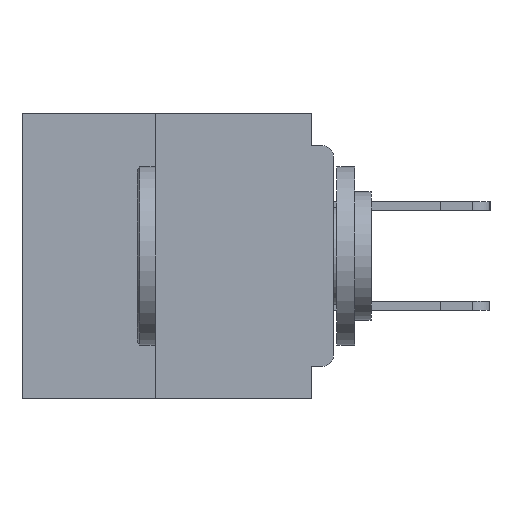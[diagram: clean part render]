
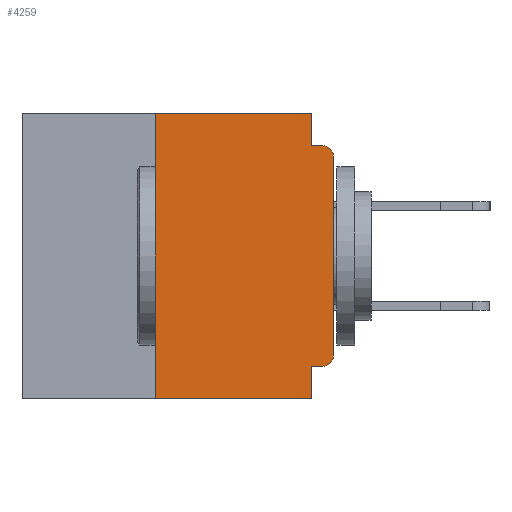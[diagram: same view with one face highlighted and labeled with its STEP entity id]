
A CAD part, left-side view. The second image highlights one B-rep face of the part: STEP entity #4259.
In plain terms, the highlighted planar face has unit normal (-1, 0, 0).
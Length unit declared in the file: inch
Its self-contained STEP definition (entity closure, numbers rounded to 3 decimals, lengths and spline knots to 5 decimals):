
#258 = AXIS2_PLACEMENT_3D ( 'NONE', #18743, #47326, #22875 ) ;
#259 = ORIENTED_EDGE ( 'NONE', *, *, #43609, .F. ) ;
#722 = DIRECTION ( 'NONE',  ( 0., 0., -1. ) ) ;
#890 = CARTESIAN_POINT ( 'NONE',  ( 0., 0.25, -0.4 ) ) ;
#1025 = LINE ( 'NONE', #19762, #39483 ) ;
#1196 = DIRECTION ( 'NONE',  ( 0., 0., -1. ) ) ;
#2159 = VERTEX_POINT ( 'NONE', #35786 ) ;
#2921 = LINE ( 'NONE', #14245, #35593 ) ;
#4256 = ORIENTED_EDGE ( 'NONE', *, *, #52456, .T. ) ;
#4259 = ADVANCED_FACE ( 'NONE', ( #37608 ), #41574, .F. ) ;
#6706 = CARTESIAN_POINT ( 'NONE',  ( 0., 0., -0.06 ) ) ;
#6852 = EDGE_CURVE ( 'NONE', #24654, #2159, #17384, .T. ) ;
#7343 = LINE ( 'NONE', #21171, #49592 ) ;
#9347 = CARTESIAN_POINT ( 'NONE',  ( 0., 0., -0.34 ) ) ;
#9559 = VERTEX_POINT ( 'NONE', #39944 ) ;
#9707 = LINE ( 'NONE', #12195, #41114 ) ;
#10303 = LINE ( 'NONE', #21649, #19936 ) ;
#10613 = EDGE_CURVE ( 'NONE', #16969, #31939, #20406, .T. ) ;
#11067 = CIRCLE ( 'NONE', #12804, 0.015 ) ;
#12195 = CARTESIAN_POINT ( 'NONE',  ( 0., 0., 0. ) ) ;
#12804 = AXIS2_PLACEMENT_3D ( 'NONE', #24137, #52662, #28261 ) ;
#14245 = CARTESIAN_POINT ( 'NONE',  ( 0., 0., -0.045 ) ) ;
#15128 = EDGE_CURVE ( 'NONE', #24654, #36146, #7343, .T. ) ;
#16969 = VERTEX_POINT ( 'NONE', #49732 ) ;
#17325 = ORIENTED_EDGE ( 'NONE', *, *, #39891, .F. ) ;
#17351 = CARTESIAN_POINT ( 'NONE',  ( 0., 0.25, -0.4 ) ) ;
#17384 = LINE ( 'NONE', #17351, #27018 ) ;
#18606 = VECTOR ( 'NONE', #28648, 39.37008 ) ;
#18615 = CARTESIAN_POINT ( 'NONE',  ( 0., 0.437, 0. ) ) ;
#18743 = CARTESIAN_POINT ( 'NONE',  ( 0., 0.015, -0.34 ) ) ;
#19762 = CARTESIAN_POINT ( 'NONE',  ( 0., 0., -0.355 ) ) ;
#19936 = VECTOR ( 'NONE', #1196, 39.37008 ) ;
#20406 = CIRCLE ( 'NONE', #258, 0.015 ) ;
#20956 = VERTEX_POINT ( 'NONE', #41401 ) ;
#21171 = CARTESIAN_POINT ( 'NONE',  ( 0., 0.437, -0.4 ) ) ;
#21241 = VERTEX_POINT ( 'NONE', #22599 ) ;
#21649 = CARTESIAN_POINT ( 'NONE',  ( 0., 0.031, 0. ) ) ;
#22599 = CARTESIAN_POINT ( 'NONE',  ( 0., 0.015, -0.045 ) ) ;
#22666 = CARTESIAN_POINT ( 'NONE',  ( 0., 0.031, -0.4 ) ) ;
#22742 = DIRECTION ( 'NONE',  ( 0., -1., 0. ) ) ;
#22875 = DIRECTION ( 'NONE',  ( 0., 0., -1. ) ) ;
#24137 = CARTESIAN_POINT ( 'NONE',  ( 0., 0.015, -0.06 ) ) ;
#24534 = CARTESIAN_POINT ( 'NONE',  ( 0., 0.031, -0.4 ) ) ;
#24654 = VERTEX_POINT ( 'NONE', #890 ) ;
#25281 = DIRECTION ( 'NONE',  ( 0., -1., 0. ) ) ;
#25291 = DIRECTION ( 'NONE',  ( 1., 0., 0. ) ) ;
#25374 = ORIENTED_EDGE ( 'NONE', *, *, #27102, .T. ) ;
#25577 = VERTEX_POINT ( 'NONE', #6706 ) ;
#27018 = VECTOR ( 'NONE', #37937, 39.37008 ) ;
#27102 = EDGE_CURVE ( 'NONE', #25577, #21241, #11067, .T. ) ;
#27140 = LINE ( 'NONE', #18615, #47571 ) ;
#27213 = AXIS2_PLACEMENT_3D ( 'NONE', #45669, #25291, #722 ) ;
#28261 = DIRECTION ( 'NONE',  ( 0., 0., -1. ) ) ;
#28648 = DIRECTION ( 'NONE',  ( 0., 0., -1. ) ) ;
#30349 = ORIENTED_EDGE ( 'NONE', *, *, #50854, .F. ) ;
#31939 = VERTEX_POINT ( 'NONE', #9347 ) ;
#32654 = ORIENTED_EDGE ( 'NONE', *, *, #45487, .F. ) ;
#33339 = EDGE_LOOP ( 'NONE', ( #4256, #25374, #17325, #259, #30349, #49176, #51919, #51648, #32654, #40803 ) ) ;
#35593 = VECTOR ( 'NONE', #38755, 39.37008 ) ;
#35786 = CARTESIAN_POINT ( 'NONE',  ( 0., 0.25, 0. ) ) ;
#36146 = VERTEX_POINT ( 'NONE', #22666 ) ;
#37086 = EDGE_CURVE ( 'NONE', #43751, #36146, #52453, .T. ) ;
#37608 = FACE_OUTER_BOUND ( 'NONE', #33339, .T. ) ;
#37937 = DIRECTION ( 'NONE',  ( 0., 0., 1. ) ) ;
#38755 = DIRECTION ( 'NONE',  ( 0., -1., 0. ) ) ;
#39483 = VECTOR ( 'NONE', #52404, 39.37008 ) ;
#39891 = EDGE_CURVE ( 'NONE', #20956, #21241, #2921, .T. ) ;
#39944 = CARTESIAN_POINT ( 'NONE',  ( 0., 0.031, 0. ) ) ;
#40803 = ORIENTED_EDGE ( 'NONE', *, *, #10613, .T. ) ;
#41114 = VECTOR ( 'NONE', #48832, 39.37008 ) ;
#41401 = CARTESIAN_POINT ( 'NONE',  ( 0., 0.031, -0.045 ) ) ;
#41574 = PLANE ( 'NONE',  #27213 ) ;
#42957 = CARTESIAN_POINT ( 'NONE',  ( 0., 0.031, -0.355 ) ) ;
#43609 = EDGE_CURVE ( 'NONE', #9559, #20956, #10303, .T. ) ;
#43751 = VERTEX_POINT ( 'NONE', #42957 ) ;
#45487 = EDGE_CURVE ( 'NONE', #16969, #43751, #1025, .T. ) ;
#45669 = CARTESIAN_POINT ( 'NONE',  ( 0., 0.437, 0. ) ) ;
#47326 = DIRECTION ( 'NONE',  ( -1., 0., 0. ) ) ;
#47571 = VECTOR ( 'NONE', #22742, 39.37008 ) ;
#48832 = DIRECTION ( 'NONE',  ( 0., 0., 1. ) ) ;
#49176 = ORIENTED_EDGE ( 'NONE', *, *, #6852, .F. ) ;
#49592 = VECTOR ( 'NONE', #25281, 39.37008 ) ;
#49732 = CARTESIAN_POINT ( 'NONE',  ( 0., 0.015, -0.355 ) ) ;
#50854 = EDGE_CURVE ( 'NONE', #2159, #9559, #27140, .T. ) ;
#51648 = ORIENTED_EDGE ( 'NONE', *, *, #37086, .F. ) ;
#51919 = ORIENTED_EDGE ( 'NONE', *, *, #15128, .T. ) ;
#52404 = DIRECTION ( 'NONE',  ( 0., 1., 0. ) ) ;
#52453 = LINE ( 'NONE', #24534, #18606 ) ;
#52456 = EDGE_CURVE ( 'NONE', #31939, #25577, #9707, .T. ) ;
#52662 = DIRECTION ( 'NONE',  ( -1., 0., 0. ) ) ;
